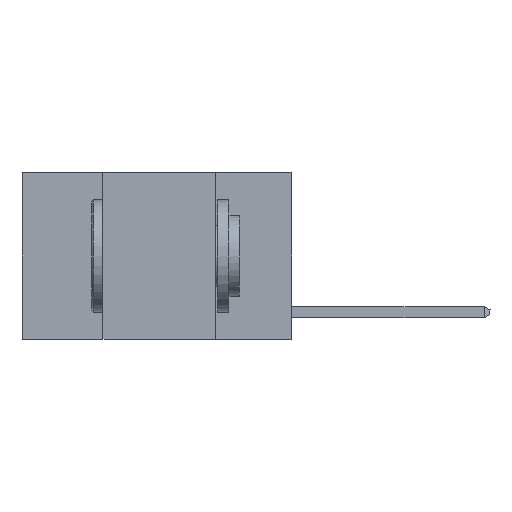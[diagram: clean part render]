
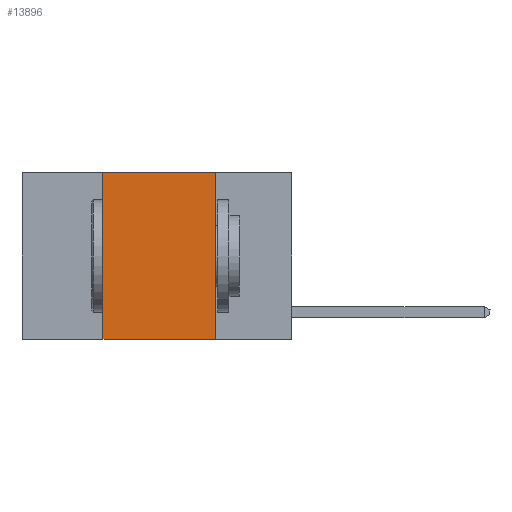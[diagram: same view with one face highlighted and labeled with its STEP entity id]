
A CAD part, left-side view. The second image highlights one B-rep face of the part: STEP entity #13896.
In plain terms, the highlighted planar face has unit normal (-1, 0, 0).
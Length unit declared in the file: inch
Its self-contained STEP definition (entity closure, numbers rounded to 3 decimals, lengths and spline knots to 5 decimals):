
#1063 = EDGE_CURVE ( 'NONE', #6114, #16714, #10155, .T. ) ;
#1122 = DIRECTION ( 'NONE',  ( 0., -1., 0. ) ) ;
#1460 = LINE ( 'NONE', #2597, #12448 ) ;
#1668 = EDGE_CURVE ( 'NONE', #16714, #17796, #11275, .T. ) ;
#1683 = VECTOR ( 'NONE', #7251, 39.37008 ) ;
#2357 = ORIENTED_EDGE ( 'NONE', *, *, #17574, .F. ) ;
#2597 = CARTESIAN_POINT ( 'NONE',  ( 0., 0.6, -0.37 ) ) ;
#3437 = ORIENTED_EDGE ( 'NONE', *, *, #8381, .T. ) ;
#4161 = DIRECTION ( 'NONE',  ( 0., 0., -1. ) ) ;
#4552 = VERTEX_POINT ( 'NONE', #10419 ) ;
#5621 = ORIENTED_EDGE ( 'NONE', *, *, #1668, .F. ) ;
#6114 = VERTEX_POINT ( 'NONE', #6359 ) ;
#6212 = LINE ( 'NONE', #7686, #7423 ) ;
#6359 = CARTESIAN_POINT ( 'NONE',  ( 0., 0.42, -0.37 ) ) ;
#7251 = DIRECTION ( 'NONE',  ( 0., 0., 1. ) ) ;
#7423 = VECTOR ( 'NONE', #12095, 39.37008 ) ;
#7686 = CARTESIAN_POINT ( 'NONE',  ( 0., 0.17, 0. ) ) ;
#8381 = EDGE_CURVE ( 'NONE', #6114, #4552, #1460, .T. ) ;
#8544 = DIRECTION ( 'NONE',  ( 0., -1., 0. ) ) ;
#9993 = FACE_OUTER_BOUND ( 'NONE', #15165, .T. ) ;
#10155 = LINE ( 'NONE', #16004, #1683 ) ;
#10168 = CARTESIAN_POINT ( 'NONE',  ( 0., 0.17, 0. ) ) ;
#10419 = CARTESIAN_POINT ( 'NONE',  ( 0., 0.17, -0.37 ) ) ;
#11275 = LINE ( 'NONE', #14357, #19018 ) ;
#11526 = DIRECTION ( 'NONE',  ( 1., 0., 0. ) ) ;
#12095 = DIRECTION ( 'NONE',  ( 0., 0., -1. ) ) ;
#12448 = VECTOR ( 'NONE', #8544, 39.37008 ) ;
#12965 = CARTESIAN_POINT ( 'NONE',  ( 0., 0.6, 0. ) ) ;
#13239 = CARTESIAN_POINT ( 'NONE',  ( 0., 0.42, 0. ) ) ;
#13896 = ADVANCED_FACE ( 'NONE', ( #9993 ), #15846, .F. ) ;
#14070 = AXIS2_PLACEMENT_3D ( 'NONE', #12965, #11526, #4161 ) ;
#14357 = CARTESIAN_POINT ( 'NONE',  ( 0., 0.6, 0. ) ) ;
#15165 = EDGE_LOOP ( 'NONE', ( #2357, #5621, #17261, #3437 ) ) ;
#15846 = PLANE ( 'NONE',  #14070 ) ;
#16004 = CARTESIAN_POINT ( 'NONE',  ( 0., 0.42, 0. ) ) ;
#16714 = VERTEX_POINT ( 'NONE', #13239 ) ;
#17261 = ORIENTED_EDGE ( 'NONE', *, *, #1063, .F. ) ;
#17574 = EDGE_CURVE ( 'NONE', #17796, #4552, #6212, .T. ) ;
#17796 = VERTEX_POINT ( 'NONE', #10168 ) ;
#19018 = VECTOR ( 'NONE', #1122, 39.37008 ) ;
